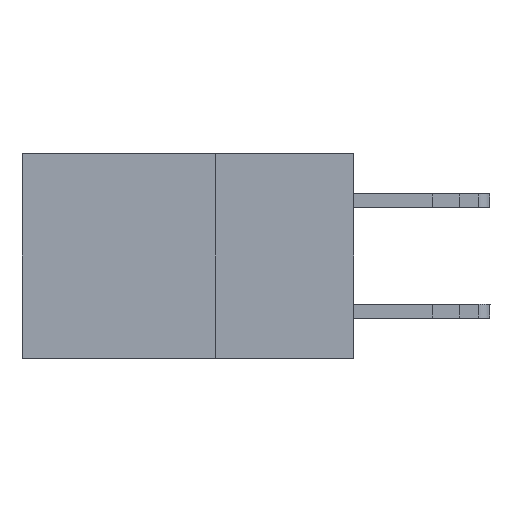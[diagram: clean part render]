
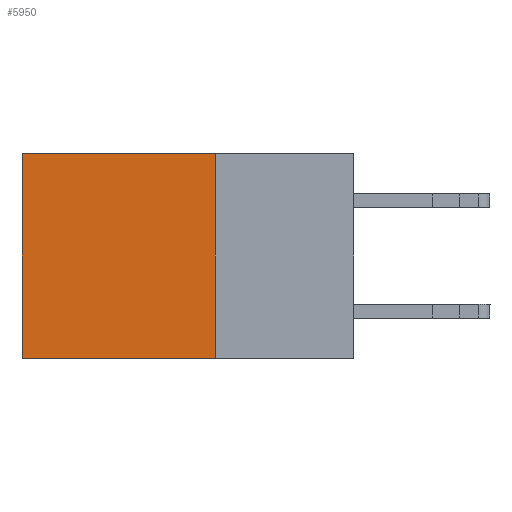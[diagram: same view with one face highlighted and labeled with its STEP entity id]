
A CAD part, left-side view. The second image highlights one B-rep face of the part: STEP entity #5950.
In plain terms, the highlighted planar face has unit normal (-1, 0, 0).
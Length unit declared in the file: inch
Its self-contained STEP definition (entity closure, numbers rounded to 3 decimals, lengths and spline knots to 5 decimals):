
#1044 = DIRECTION ( 'NONE',  ( 1., 0., 0. ) ) ;
#3028 = CARTESIAN_POINT ( 'NONE',  ( 0.2875, 0.25, 0. ) ) ;
#3534 = LINE ( 'NONE', #12544, #18255 ) ;
#3666 = LINE ( 'NONE', #13167, #12759 ) ;
#3918 = VERTEX_POINT ( 'NONE', #18211 ) ;
#3977 = FACE_OUTER_BOUND ( 'NONE', #14184, .T. ) ;
#4535 = LINE ( 'NONE', #3028, #6851 ) ;
#4907 = EDGE_CURVE ( 'NONE', #5220, #17400, #16334, .T. ) ;
#5220 = VERTEX_POINT ( 'NONE', #14482 ) ;
#5950 = ADVANCED_FACE ( 'NONE', ( #3977 ), #10093, .F. ) ;
#6851 = VECTOR ( 'NONE', #9151, 39.37008 ) ;
#7377 = VECTOR ( 'NONE', #18013, 39.37008 ) ;
#7969 = EDGE_CURVE ( 'NONE', #3918, #17400, #3534, .T. ) ;
#9151 = DIRECTION ( 'NONE',  ( 0., 1., 0. ) ) ;
#9471 = CARTESIAN_POINT ( 'NONE',  ( 0.2875, 0.25, 0. ) ) ;
#9632 = DIRECTION ( 'NONE',  ( 0., 1., 0. ) ) ;
#9956 = AXIS2_PLACEMENT_3D ( 'NONE', #16192, #1044, #14971 ) ;
#10093 = PLANE ( 'NONE',  #9956 ) ;
#10149 = CARTESIAN_POINT ( 'NONE',  ( 0.2875, 0.6, 0. ) ) ;
#10862 = ORIENTED_EDGE ( 'NONE', *, *, #18141, .T. ) ;
#12317 = CARTESIAN_POINT ( 'NONE',  ( 0.2875, 0.6, -0.37 ) ) ;
#12544 = CARTESIAN_POINT ( 'NONE',  ( 0.2875, 0.25, -0.37 ) ) ;
#12759 = VECTOR ( 'NONE', #17758, 39.37008 ) ;
#13167 = CARTESIAN_POINT ( 'NONE',  ( 0.2875, 0.25, 0. ) ) ;
#14184 = EDGE_LOOP ( 'NONE', ( #17935, #17591, #18075, #10862 ) ) ;
#14482 = CARTESIAN_POINT ( 'NONE',  ( 0.2875, 0.6, 0. ) ) ;
#14971 = DIRECTION ( 'NONE',  ( 0., 0., -1. ) ) ;
#15322 = VERTEX_POINT ( 'NONE', #9471 ) ;
#16192 = CARTESIAN_POINT ( 'NONE',  ( 0.2875, 0.25, 0. ) ) ;
#16334 = LINE ( 'NONE', #10149, #7377 ) ;
#17400 = VERTEX_POINT ( 'NONE', #12317 ) ;
#17591 = ORIENTED_EDGE ( 'NONE', *, *, #7969, .F. ) ;
#17758 = DIRECTION ( 'NONE',  ( 0., 0., -1. ) ) ;
#17935 = ORIENTED_EDGE ( 'NONE', *, *, #4907, .T. ) ;
#18013 = DIRECTION ( 'NONE',  ( 0., 0., -1. ) ) ;
#18075 = ORIENTED_EDGE ( 'NONE', *, *, #18958, .F. ) ;
#18141 = EDGE_CURVE ( 'NONE', #15322, #5220, #4535, .T. ) ;
#18211 = CARTESIAN_POINT ( 'NONE',  ( 0.2875, 0.25, -0.37 ) ) ;
#18255 = VECTOR ( 'NONE', #9632, 39.37008 ) ;
#18958 = EDGE_CURVE ( 'NONE', #15322, #3918, #3666, .T. ) ;
